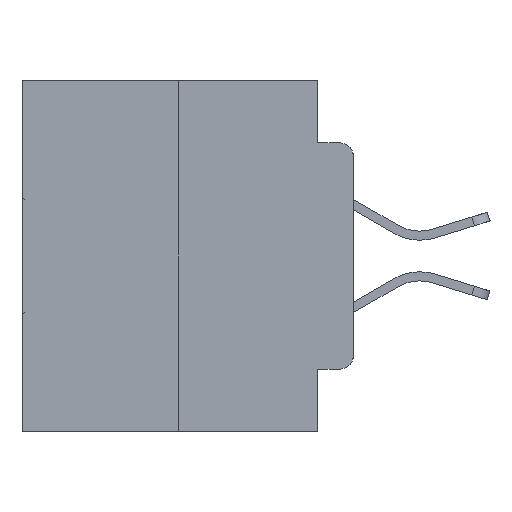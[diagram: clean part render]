
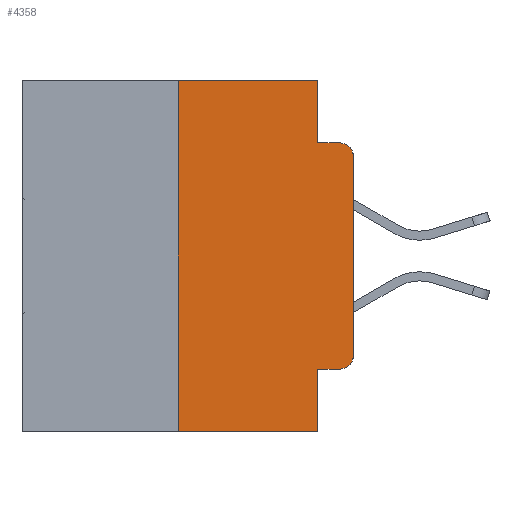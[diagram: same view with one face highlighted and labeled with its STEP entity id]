
A CAD part, left-side view. The second image highlights one B-rep face of the part: STEP entity #4358.
In plain terms, the highlighted planar face has unit normal (-1, 0, 0).
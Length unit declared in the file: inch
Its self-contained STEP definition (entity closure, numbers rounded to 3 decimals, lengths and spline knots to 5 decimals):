
#84 = EDGE_CURVE ( 'NONE', #3688, #22095, #16303, .T. ) ;
#155 = CARTESIAN_POINT ( 'NONE',  ( 0., 0., 0. ) ) ;
#1017 = EDGE_CURVE ( 'NONE', #15587, #20750, #6994, .T. ) ;
#1740 = VECTOR ( 'NONE', #9205, 39.37008 ) ;
#1840 = VERTEX_POINT ( 'NONE', #5100 ) ;
#2157 = AXIS2_PLACEMENT_3D ( 'NONE', #16550, #25614, #12383 ) ;
#2478 = ORIENTED_EDGE ( 'NONE', *, *, #3861, .F. ) ;
#3557 = CARTESIAN_POINT ( 'NONE',  ( 0., 0., -0.3915 ) ) ;
#3688 = VERTEX_POINT ( 'NONE', #25924 ) ;
#3706 = DIRECTION ( 'NONE',  ( 0., 0., -1. ) ) ;
#3767 = CARTESIAN_POINT ( 'NONE',  ( 0., 0.473, 0. ) ) ;
#3861 = EDGE_CURVE ( 'NONE', #3688, #1840, #19822, .T. ) ;
#4358 = ADVANCED_FACE ( 'NONE', ( #12083 ), #21158, .F. ) ;
#4547 = DIRECTION ( 'NONE',  ( 0., 0., -1. ) ) ;
#4567 = DIRECTION ( 'NONE',  ( 0., -1., 0. ) ) ;
#5100 = CARTESIAN_POINT ( 'NONE',  ( 0., 0.051, -0.5 ) ) ;
#5155 = CARTESIAN_POINT ( 'NONE',  ( 0., 0.051, 0. ) ) ;
#6590 = EDGE_CURVE ( 'NONE', #20750, #27944, #14254, .T. ) ;
#6954 = LINE ( 'NONE', #16046, #1740 ) ;
#6994 = LINE ( 'NONE', #16077, #7620 ) ;
#7620 = VECTOR ( 'NONE', #28408, 39.37008 ) ;
#7768 = EDGE_CURVE ( 'NONE', #15587, #1840, #6954, .T. ) ;
#8630 = AXIS2_PLACEMENT_3D ( 'NONE', #24962, #26760, #4547 ) ;
#8825 = CARTESIAN_POINT ( 'NONE',  ( 0., 0.02, -0.3915 ) ) ;
#9006 = VECTOR ( 'NONE', #4567, 39.37008 ) ;
#9205 = DIRECTION ( 'NONE',  ( 0., -1., 0. ) ) ;
#9739 = DIRECTION ( 'NONE',  ( 0., -1., 0. ) ) ;
#10185 = VECTOR ( 'NONE', #9739, 39.37008 ) ;
#10220 = DIRECTION ( 'NONE',  ( 0., -1., 0. ) ) ;
#10284 = ORIENTED_EDGE ( 'NONE', *, *, #14158, .T. ) ;
#10823 = ORIENTED_EDGE ( 'NONE', *, *, #7768, .T. ) ;
#11240 = ORIENTED_EDGE ( 'NONE', *, *, #6590, .F. ) ;
#11745 = LINE ( 'NONE', #5155, #13867 ) ;
#12083 = FACE_OUTER_BOUND ( 'NONE', #16878, .T. ) ;
#12383 = DIRECTION ( 'NONE',  ( 0., 0., -1. ) ) ;
#12681 = CARTESIAN_POINT ( 'NONE',  ( 0., 0.051, 0. ) ) ;
#13867 = VECTOR ( 'NONE', #20526, 39.37008 ) ;
#13903 = CIRCLE ( 'NONE', #8630, 0.02 ) ;
#14158 = EDGE_CURVE ( 'NONE', #23886, #27285, #13903, .T. ) ;
#14196 = DIRECTION ( 'NONE',  ( 0., 0., 1. ) ) ;
#14254 = LINE ( 'NONE', #3767, #22151 ) ;
#14578 = ORIENTED_EDGE ( 'NONE', *, *, #28008, .F. ) ;
#14869 = AXIS2_PLACEMENT_3D ( 'NONE', #8825, #17912, #26976 ) ;
#15068 = CARTESIAN_POINT ( 'NONE',  ( 0., 0., -0.1085 ) ) ;
#15587 = VERTEX_POINT ( 'NONE', #25407 ) ;
#16046 = CARTESIAN_POINT ( 'NONE',  ( 0., 0.473, -0.5 ) ) ;
#16077 = CARTESIAN_POINT ( 'NONE',  ( 0., 0.25, 0. ) ) ;
#16303 = LINE ( 'NONE', #23267, #10185 ) ;
#16324 = EDGE_CURVE ( 'NONE', #22095, #17239, #17716, .T. ) ;
#16363 = CARTESIAN_POINT ( 'NONE',  ( 0., 0.051, 0. ) ) ;
#16550 = CARTESIAN_POINT ( 'NONE',  ( 0., 0.473, 0. ) ) ;
#16878 = EDGE_LOOP ( 'NONE', ( #18195, #10284, #20164, #14578, #11240, #24643, #10823, #2478, #23864, #23083 ) ) ;
#17239 = VERTEX_POINT ( 'NONE', #3557 ) ;
#17716 = CIRCLE ( 'NONE', #14869, 0.02 ) ;
#17912 = DIRECTION ( 'NONE',  ( -1., 0., 0. ) ) ;
#18108 = CARTESIAN_POINT ( 'NONE',  ( 0., 0.25, 0. ) ) ;
#18195 = ORIENTED_EDGE ( 'NONE', *, *, #23679, .T. ) ;
#19822 = LINE ( 'NONE', #12681, #24111 ) ;
#20164 = ORIENTED_EDGE ( 'NONE', *, *, #24541, .F. ) ;
#20377 = CARTESIAN_POINT ( 'NONE',  ( 0., 0.051, -0.0885 ) ) ;
#20526 = DIRECTION ( 'NONE',  ( 0., 0., -1. ) ) ;
#20677 = LINE ( 'NONE', #20377, #9006 ) ;
#20750 = VERTEX_POINT ( 'NONE', #18108 ) ;
#21034 = LINE ( 'NONE', #155, #23223 ) ;
#21158 = PLANE ( 'NONE',  #2157 ) ;
#22095 = VERTEX_POINT ( 'NONE', #23576 ) ;
#22151 = VECTOR ( 'NONE', #10220, 39.37008 ) ;
#23083 = ORIENTED_EDGE ( 'NONE', *, *, #16324, .T. ) ;
#23223 = VECTOR ( 'NONE', #14196, 39.37008 ) ;
#23267 = CARTESIAN_POINT ( 'NONE',  ( 0., 0.051, -0.4115 ) ) ;
#23576 = CARTESIAN_POINT ( 'NONE',  ( 0., 0.02, -0.4115 ) ) ;
#23679 = EDGE_CURVE ( 'NONE', #17239, #23886, #21034, .T. ) ;
#23864 = ORIENTED_EDGE ( 'NONE', *, *, #84, .T. ) ;
#23886 = VERTEX_POINT ( 'NONE', #15068 ) ;
#23955 = VERTEX_POINT ( 'NONE', #29345 ) ;
#24111 = VECTOR ( 'NONE', #3706, 39.37008 ) ;
#24541 = EDGE_CURVE ( 'NONE', #23955, #27285, #20677, .T. ) ;
#24643 = ORIENTED_EDGE ( 'NONE', *, *, #1017, .F. ) ;
#24962 = CARTESIAN_POINT ( 'NONE',  ( 0., 0.02, -0.1085 ) ) ;
#25407 = CARTESIAN_POINT ( 'NONE',  ( 0., 0.25, -0.5 ) ) ;
#25614 = DIRECTION ( 'NONE',  ( 1., 0., 0. ) ) ;
#25924 = CARTESIAN_POINT ( 'NONE',  ( 0., 0.051, -0.4115 ) ) ;
#26760 = DIRECTION ( 'NONE',  ( -1., 0., 0. ) ) ;
#26976 = DIRECTION ( 'NONE',  ( 0., 0., -1. ) ) ;
#27285 = VERTEX_POINT ( 'NONE', #29346 ) ;
#27944 = VERTEX_POINT ( 'NONE', #16363 ) ;
#28008 = EDGE_CURVE ( 'NONE', #27944, #23955, #11745, .T. ) ;
#28408 = DIRECTION ( 'NONE',  ( 0., 0., 1. ) ) ;
#29345 = CARTESIAN_POINT ( 'NONE',  ( 0., 0.051, -0.0885 ) ) ;
#29346 = CARTESIAN_POINT ( 'NONE',  ( 0., 0.02, -0.0885 ) ) ;
